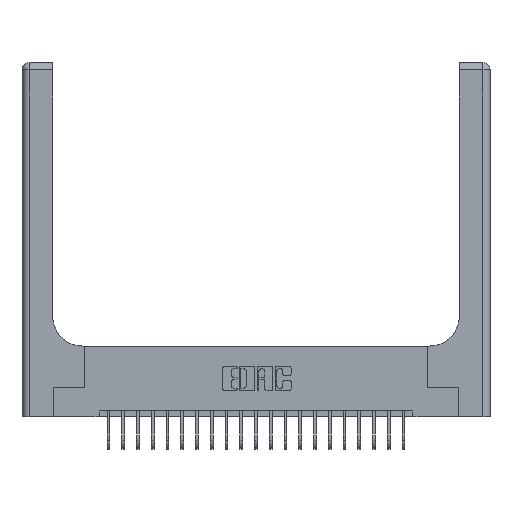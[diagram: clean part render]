
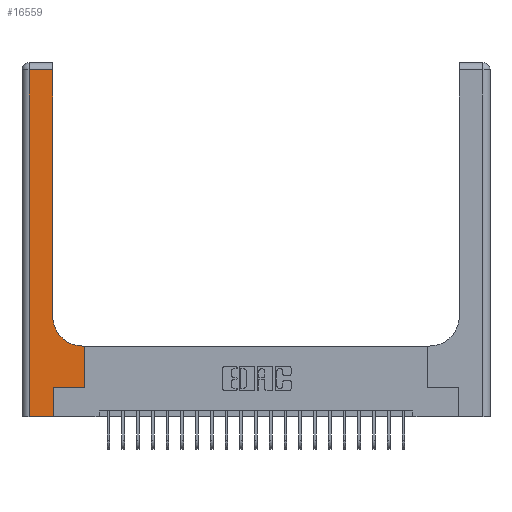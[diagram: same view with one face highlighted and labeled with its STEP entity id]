
A CAD part, top view. The second image highlights one B-rep face of the part: STEP entity #16559.
In plain terms, the highlighted planar face has unit normal (0, 0, 1).
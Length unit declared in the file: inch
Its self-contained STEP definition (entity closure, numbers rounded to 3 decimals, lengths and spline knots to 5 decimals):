
#495 = EDGE_CURVE ( 'NONE', #7245, #13513, #8055, .T. ) ;
#514 = VECTOR ( 'NONE', #20099, 39.37008 ) ;
#1129 = LINE ( 'NONE', #12425, #17963 ) ;
#1257 = CARTESIAN_POINT ( 'NONE',  ( 0.265, 0., 0.37 ) ) ;
#1383 = EDGE_CURVE ( 'NONE', #20239, #2098, #7601, .T. ) ;
#1387 = CARTESIAN_POINT ( 'NONE',  ( 0.26, 2.94, 0.37 ) ) ;
#1405 = EDGE_CURVE ( 'NONE', #6393, #7245, #6484, .T. ) ;
#1808 = AXIS2_PLACEMENT_3D ( 'NONE', #12692, #9352, #11082 ) ;
#2098 = VERTEX_POINT ( 'NONE', #16065 ) ;
#2182 = LINE ( 'NONE', #6653, #13288 ) ;
#2700 = FACE_OUTER_BOUND ( 'NONE', #7386, .T. ) ;
#3583 = ORIENTED_EDGE ( 'NONE', *, *, #1405, .T. ) ;
#4204 = EDGE_CURVE ( 'NONE', #5360, #20239, #2182, .T. ) ;
#4234 = ORIENTED_EDGE ( 'NONE', *, *, #1383, .T. ) ;
#4807 = CARTESIAN_POINT ( 'NONE',  ( 0.26, 0.6, 0.37 ) ) ;
#4962 = DIRECTION ( 'NONE',  ( 0., 1., 0. ) ) ;
#5082 = CARTESIAN_POINT ( 'NONE',  ( 0.528, 0.25, 0.37 ) ) ;
#5333 = LINE ( 'NONE', #9333, #19584 ) ;
#5360 = VERTEX_POINT ( 'NONE', #17321 ) ;
#5865 = ORIENTED_EDGE ( 'NONE', *, *, #16884, .T. ) ;
#6130 = VECTOR ( 'NONE', #12546, 39.37008 ) ;
#6347 = AXIS2_PLACEMENT_3D ( 'NONE', #15998, #20601, #15678 ) ;
#6393 = VERTEX_POINT ( 'NONE', #6750 ) ;
#6484 = LINE ( 'NONE', #5082, #21444 ) ;
#6653 = CARTESIAN_POINT ( 'NONE',  ( 0., 0., 0.37 ) ) ;
#6750 = CARTESIAN_POINT ( 'NONE',  ( 0.528, 0.25, 0.37 ) ) ;
#7245 = VERTEX_POINT ( 'NONE', #17473 ) ;
#7266 = ORIENTED_EDGE ( 'NONE', *, *, #495, .T. ) ;
#7386 = EDGE_LOOP ( 'NONE', ( #5865, #20941, #16079, #8649, #4234, #15641, #3583, #7266, #18854 ) ) ;
#7601 = LINE ( 'NONE', #1257, #6130 ) ;
#8055 = LINE ( 'NONE', #4807, #20390 ) ;
#8164 = DIRECTION ( 'NONE',  ( -1., 0., 0. ) ) ;
#8649 = ORIENTED_EDGE ( 'NONE', *, *, #4204, .T. ) ;
#8769 = CIRCLE ( 'NONE', #6347, 0.25 ) ;
#9333 = CARTESIAN_POINT ( 'NONE',  ( 0.26, 3., 0.37 ) ) ;
#9352 = DIRECTION ( 'NONE',  ( 0., 0., -1. ) ) ;
#10031 = CARTESIAN_POINT ( 'NONE',  ( 0., 2.94, 0.37 ) ) ;
#10097 = CARTESIAN_POINT ( 'NONE',  ( 0.265, 0., 0.37 ) ) ;
#10188 = CARTESIAN_POINT ( 'NONE',  ( 0.06, 2.94, 0.37 ) ) ;
#10809 = DIRECTION ( 'NONE',  ( 0., -1., 0. ) ) ;
#11082 = DIRECTION ( 'NONE',  ( -1., 0., 0. ) ) ;
#11395 = VERTEX_POINT ( 'NONE', #10188 ) ;
#12058 = EDGE_CURVE ( 'NONE', #11395, #5360, #1129, .T. ) ;
#12374 = PLANE ( 'NONE',  #1808 ) ;
#12425 = CARTESIAN_POINT ( 'NONE',  ( 0.06, 3., 0.37 ) ) ;
#12546 = DIRECTION ( 'NONE',  ( 0., 1., 0. ) ) ;
#12692 = CARTESIAN_POINT ( 'NONE',  ( 0., 3., 0.37 ) ) ;
#13288 = VECTOR ( 'NONE', #20092, 39.37008 ) ;
#13397 = LINE ( 'NONE', #10031, #514 ) ;
#13513 = VERTEX_POINT ( 'NONE', #15400 ) ;
#14307 = VECTOR ( 'NONE', #21461, 39.37008 ) ;
#14781 = CARTESIAN_POINT ( 'NONE',  ( 0.265, 0.25, 0.37 ) ) ;
#15309 = EDGE_CURVE ( 'NONE', #15907, #11395, #13397, .T. ) ;
#15400 = CARTESIAN_POINT ( 'NONE',  ( 0.51, 0.6, 0.37 ) ) ;
#15641 = ORIENTED_EDGE ( 'NONE', *, *, #16680, .T. ) ;
#15678 = DIRECTION ( 'NONE',  ( 1., 0., 0. ) ) ;
#15907 = VERTEX_POINT ( 'NONE', #1387 ) ;
#15998 = CARTESIAN_POINT ( 'NONE',  ( 0.51, 0.85, 0.37 ) ) ;
#16065 = CARTESIAN_POINT ( 'NONE',  ( 0.265, 0.25, 0.37 ) ) ;
#16079 = ORIENTED_EDGE ( 'NONE', *, *, #12058, .T. ) ;
#16476 = EDGE_CURVE ( 'NONE', #13513, #19446, #8769, .T. ) ;
#16559 = ADVANCED_FACE ( 'NONE', ( #2700 ), #12374, .F. ) ;
#16680 = EDGE_CURVE ( 'NONE', #2098, #6393, #19597, .T. ) ;
#16884 = EDGE_CURVE ( 'NONE', #19446, #15907, #5333, .T. ) ;
#17321 = CARTESIAN_POINT ( 'NONE',  ( 0.06, 0., 0.37 ) ) ;
#17473 = CARTESIAN_POINT ( 'NONE',  ( 0.528, 0.6, 0.37 ) ) ;
#17963 = VECTOR ( 'NONE', #10809, 39.37008 ) ;
#18854 = ORIENTED_EDGE ( 'NONE', *, *, #16476, .T. ) ;
#18855 = CARTESIAN_POINT ( 'NONE',  ( 0.26, 0.85, 0.37 ) ) ;
#19259 = DIRECTION ( 'NONE',  ( 0., 1., 0. ) ) ;
#19446 = VERTEX_POINT ( 'NONE', #18855 ) ;
#19584 = VECTOR ( 'NONE', #19259, 39.37008 ) ;
#19597 = LINE ( 'NONE', #14781, #14307 ) ;
#20092 = DIRECTION ( 'NONE',  ( 1., 0., 0. ) ) ;
#20099 = DIRECTION ( 'NONE',  ( -1., 0., 0. ) ) ;
#20239 = VERTEX_POINT ( 'NONE', #10097 ) ;
#20390 = VECTOR ( 'NONE', #8164, 39.37008 ) ;
#20601 = DIRECTION ( 'NONE',  ( 0., 0., -1. ) ) ;
#20941 = ORIENTED_EDGE ( 'NONE', *, *, #15309, .T. ) ;
#21444 = VECTOR ( 'NONE', #4962, 39.37008 ) ;
#21461 = DIRECTION ( 'NONE',  ( 1., 0., 0. ) ) ;
